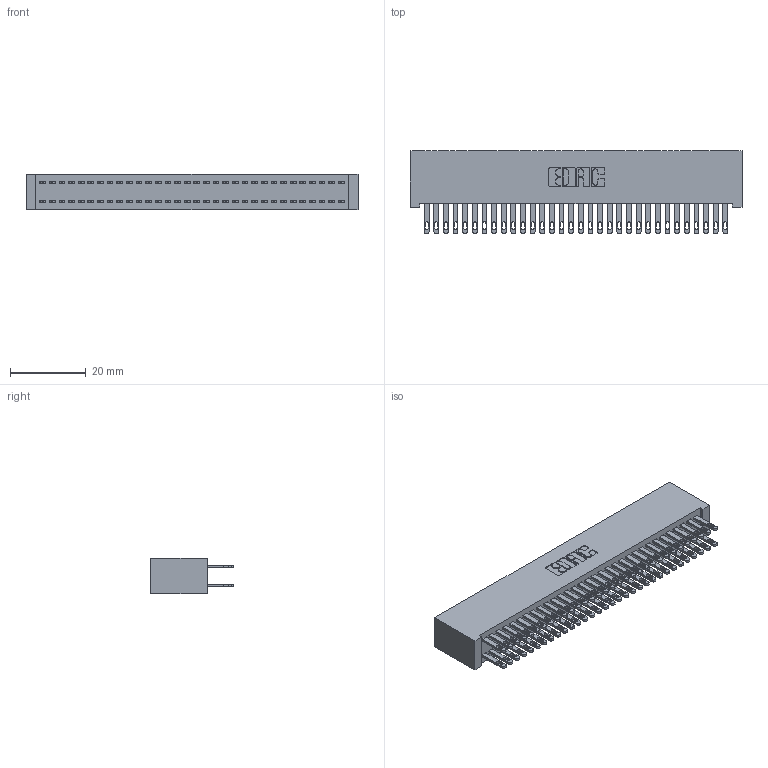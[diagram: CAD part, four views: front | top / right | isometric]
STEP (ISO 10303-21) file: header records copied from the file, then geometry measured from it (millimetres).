
FILE_DESCRIPTION (( 'STEP AP203' ), '1' );
FILE_NAME ('892-064-500-201.STEP', '2020-09-21T19:19:03', ( '' ), ( '' ), 'SwSTEP 2.0', 'SolidWorks 2020', '' );
FILE_SCHEMA (( 'CONFIG_CONTROL_DESIGN' ));
Length unit declared in the file: inch
Products named in the file (3): 892-064-500-201; 842 Part_Lugless; 345-292-001_345-293-100
Assembly tree (65 placements, depth 2):
  892-064-500-201
    842 Part_Lugless
    345-292-001_345-293-100  x64
Bounding box: 87.53 x 21.85 x 9.4 mm (x, y, z)
Volume: 8452.2 mm3; surface area: 14570.6 mm2
Topology: 65 solids, 65 shells, 3174 faces, 9683 edges, 6454 vertices
Faces by surface type: plane 1982, cylinder 1192
Entity records: 21401 total; most frequent: CARTESIAN_POINT 3554, ORIENTED_EDGE 3490, DIRECTION 3049, EDGE_CURVE 1745, VECTOR 1621, LINE 1621, VERTEX_POINT 1162, AXIS2_PLACEMENT_3D 714
